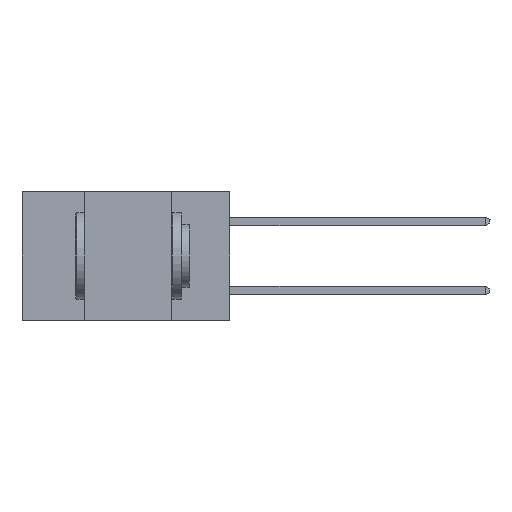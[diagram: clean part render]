
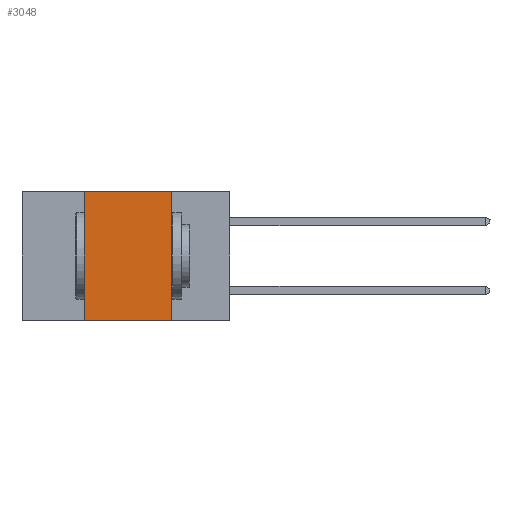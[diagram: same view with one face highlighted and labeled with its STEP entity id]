
A CAD part, left-side view. The second image highlights one B-rep face of the part: STEP entity #3048.
In plain terms, the highlighted planar face has unit normal (-1, 0, 0).
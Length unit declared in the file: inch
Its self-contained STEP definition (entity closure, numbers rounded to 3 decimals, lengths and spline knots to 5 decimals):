
#744 = EDGE_CURVE ( 'NONE', #2702, #2798, #16280, .T. ) ;
#1352 = CARTESIAN_POINT ( 'NONE',  ( 0., 0.6, -0.37 ) ) ;
#2120 = ORIENTED_EDGE ( 'NONE', *, *, #12438, .F. ) ;
#2475 = VECTOR ( 'NONE', #3458, 39.37008 ) ;
#2702 = VERTEX_POINT ( 'NONE', #12172 ) ;
#2798 = VERTEX_POINT ( 'NONE', #14244 ) ;
#3048 = ADVANCED_FACE ( 'NONE', ( #13478 ), #8879, .F. ) ;
#3458 = DIRECTION ( 'NONE',  ( 0., 0., 1. ) ) ;
#5938 = VERTEX_POINT ( 'NONE', #10762 ) ;
#6604 = CARTESIAN_POINT ( 'NONE',  ( 0., 0.42, -0.37 ) ) ;
#7232 = EDGE_CURVE ( 'NONE', #5938, #2798, #9367, .T. ) ;
#7486 = CARTESIAN_POINT ( 'NONE',  ( 0., 0.6, 0. ) ) ;
#7987 = EDGE_CURVE ( 'NONE', #2702, #14889, #8350, .T. ) ;
#8246 = EDGE_LOOP ( 'NONE', ( #14337, #2120, #17696, #11334 ) ) ;
#8350 = LINE ( 'NONE', #6604, #2475 ) ;
#8879 = PLANE ( 'NONE',  #17963 ) ;
#9367 = LINE ( 'NONE', #19065, #19518 ) ;
#10119 = CARTESIAN_POINT ( 'NONE',  ( 0., 0.42, 0. ) ) ;
#10399 = DIRECTION ( 'NONE',  ( 0., 0., -1. ) ) ;
#10762 = CARTESIAN_POINT ( 'NONE',  ( 0., 0.17, 0. ) ) ;
#11334 = ORIENTED_EDGE ( 'NONE', *, *, #744, .T. ) ;
#12146 = CARTESIAN_POINT ( 'NONE',  ( 0., 0.6, 0. ) ) ;
#12172 = CARTESIAN_POINT ( 'NONE',  ( 0., 0.42, -0.37 ) ) ;
#12438 = EDGE_CURVE ( 'NONE', #14889, #5938, #19031, .T. ) ;
#13478 = FACE_OUTER_BOUND ( 'NONE', #8246, .T. ) ;
#13969 = DIRECTION ( 'NONE',  ( 0., 0., -1. ) ) ;
#14014 = VECTOR ( 'NONE', #20881, 39.37008 ) ;
#14244 = CARTESIAN_POINT ( 'NONE',  ( 0., 0.17, -0.37 ) ) ;
#14337 = ORIENTED_EDGE ( 'NONE', *, *, #7232, .F. ) ;
#14889 = VERTEX_POINT ( 'NONE', #10119 ) ;
#15477 = VECTOR ( 'NONE', #21278, 39.37008 ) ;
#16280 = LINE ( 'NONE', #1352, #15477 ) ;
#17696 = ORIENTED_EDGE ( 'NONE', *, *, #7987, .F. ) ;
#17963 = AXIS2_PLACEMENT_3D ( 'NONE', #12146, #20101, #10399 ) ;
#19031 = LINE ( 'NONE', #7486, #14014 ) ;
#19065 = CARTESIAN_POINT ( 'NONE',  ( 0., 0.17, -0.37 ) ) ;
#19518 = VECTOR ( 'NONE', #13969, 39.37008 ) ;
#20101 = DIRECTION ( 'NONE',  ( 1., 0., 0. ) ) ;
#20881 = DIRECTION ( 'NONE',  ( 0., -1., 0. ) ) ;
#21278 = DIRECTION ( 'NONE',  ( 0., -1., 0. ) ) ;
